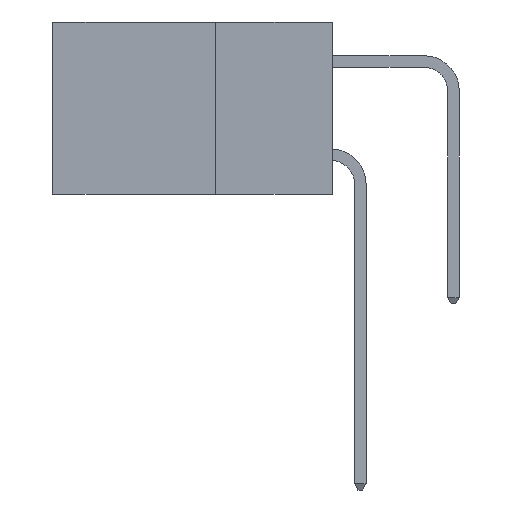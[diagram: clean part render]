
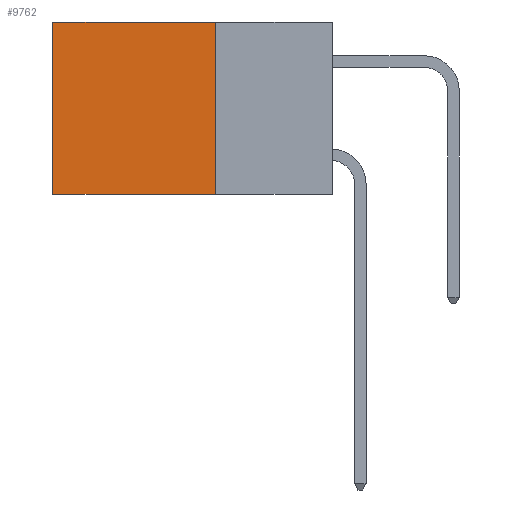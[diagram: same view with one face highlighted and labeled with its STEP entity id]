
A CAD part, left-side view. The second image highlights one B-rep face of the part: STEP entity #9762.
In plain terms, the highlighted planar face has unit normal (-1, 0, 0).
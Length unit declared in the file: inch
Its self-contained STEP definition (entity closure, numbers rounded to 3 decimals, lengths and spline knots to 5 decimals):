
#59 = CARTESIAN_POINT ( 'NONE',  ( 0.2615, 0.25, -0.37 ) ) ;
#171 = VECTOR ( 'NONE', #13537, 39.37008 ) ;
#400 = VERTEX_POINT ( 'NONE', #12894 ) ;
#880 = EDGE_CURVE ( 'NONE', #4999, #6427, #10318, .T. ) ;
#1363 = EDGE_CURVE ( 'NONE', #400, #7834, #10748, .T. ) ;
#1657 = DIRECTION ( 'NONE',  ( 1., 0., 0. ) ) ;
#1773 = CARTESIAN_POINT ( 'NONE',  ( 0.2615, 0.6, -0.37 ) ) ;
#2375 = FACE_OUTER_BOUND ( 'NONE', #14627, .T. ) ;
#2493 = VECTOR ( 'NONE', #8314, 39.37008 ) ;
#2507 = VECTOR ( 'NONE', #9727, 39.37008 ) ;
#3198 = ORIENTED_EDGE ( 'NONE', *, *, #880, .F. ) ;
#4244 = AXIS2_PLACEMENT_3D ( 'NONE', #15432, #1657, #11377 ) ;
#4999 = VERTEX_POINT ( 'NONE', #6210 ) ;
#5641 = CARTESIAN_POINT ( 'NONE',  ( 0.2615, 0.6, -0.37 ) ) ;
#6210 = CARTESIAN_POINT ( 'NONE',  ( 0.2615, 0.25, 0. ) ) ;
#6427 = VERTEX_POINT ( 'NONE', #14644 ) ;
#6596 = LINE ( 'NONE', #59, #2493 ) ;
#7602 = ORIENTED_EDGE ( 'NONE', *, *, #1363, .T. ) ;
#7607 = EDGE_CURVE ( 'NONE', #6427, #7834, #6596, .T. ) ;
#7834 = VERTEX_POINT ( 'NONE', #1773 ) ;
#8085 = DIRECTION ( 'NONE',  ( 0., 1., 0. ) ) ;
#8236 = ORIENTED_EDGE ( 'NONE', *, *, #9016, .T. ) ;
#8314 = DIRECTION ( 'NONE',  ( 0., 1., 0. ) ) ;
#8607 = ORIENTED_EDGE ( 'NONE', *, *, #7607, .F. ) ;
#9016 = EDGE_CURVE ( 'NONE', #4999, #400, #12903, .T. ) ;
#9727 = DIRECTION ( 'NONE',  ( 0., 0., -1. ) ) ;
#9762 = ADVANCED_FACE ( 'NONE', ( #2375 ), #15498, .F. ) ;
#10318 = LINE ( 'NONE', #13895, #171 ) ;
#10748 = LINE ( 'NONE', #5641, #2507 ) ;
#10903 = CARTESIAN_POINT ( 'NONE',  ( 0.2615, 0.25, 0. ) ) ;
#11377 = DIRECTION ( 'NONE',  ( 0., 0., -1. ) ) ;
#12894 = CARTESIAN_POINT ( 'NONE',  ( 0.2615, 0.6, 0. ) ) ;
#12903 = LINE ( 'NONE', #10903, #16094 ) ;
#13537 = DIRECTION ( 'NONE',  ( 0., 0., -1. ) ) ;
#13895 = CARTESIAN_POINT ( 'NONE',  ( 0.2615, 0.25, -0.37 ) ) ;
#14627 = EDGE_LOOP ( 'NONE', ( #7602, #8607, #3198, #8236 ) ) ;
#14644 = CARTESIAN_POINT ( 'NONE',  ( 0.2615, 0.25, -0.37 ) ) ;
#15432 = CARTESIAN_POINT ( 'NONE',  ( 0.2615, 0.25, -0.37 ) ) ;
#15498 = PLANE ( 'NONE',  #4244 ) ;
#16094 = VECTOR ( 'NONE', #8085, 39.37008 ) ;
